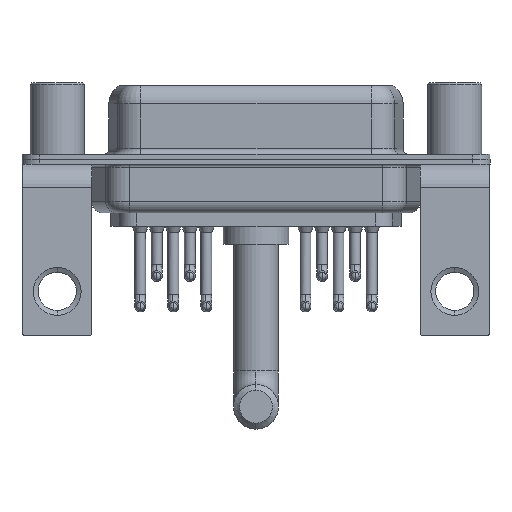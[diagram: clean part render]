
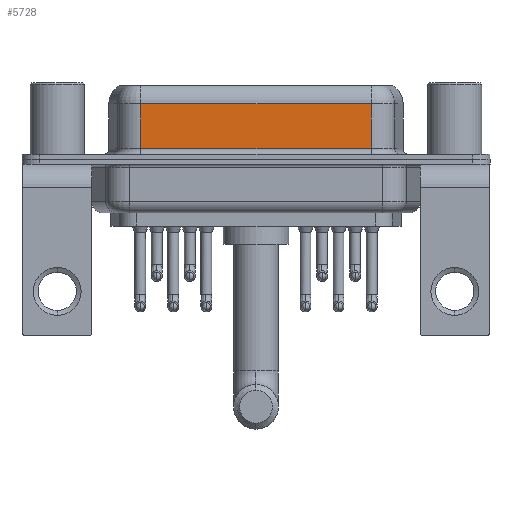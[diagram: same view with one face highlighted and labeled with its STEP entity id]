
A CAD part, front view. The second image highlights one B-rep face of the part: STEP entity #5728.
In plain terms, the highlighted planar face has unit normal (0, -1, 0).
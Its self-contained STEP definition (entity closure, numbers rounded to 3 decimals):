
#185 = LINE ( 'NONE', #8413, #10999 ) ;
#304 = AXIS2_PLACEMENT_3D ( 'NONE', #20353, #5644, #18735 ) ;
#498 = EDGE_CURVE ( 'NONE', #4229, #19295, #185, .T. ) ;
#1807 = CARTESIAN_POINT ( 'NONE',  ( 7.013, -3.95, 4.65 ) ) ;
#2610 = CARTESIAN_POINT ( 'NONE',  ( 26.287, -3.95, 4.65 ) ) ;
#3554 = LINE ( 'NONE', #11489, #19229 ) ;
#4017 = VERTEX_POINT ( 'NONE', #8275 ) ;
#4229 = VERTEX_POINT ( 'NONE', #2610 ) ;
#5076 = CARTESIAN_POINT ( 'NONE',  ( 26.287, -3.95, 4.65 ) ) ;
#5337 = CARTESIAN_POINT ( 'NONE',  ( 7.013, -3.95, 6.4 ) ) ;
#5644 = DIRECTION ( 'NONE',  ( 0., 1., 0. ) ) ;
#5728 = ADVANCED_FACE ( 'NONE', ( #13794 ), #16691, .F. ) ;
#6533 = ORIENTED_EDGE ( 'NONE', *, *, #8854, .T. ) ;
#7129 = DIRECTION ( 'NONE',  ( 0., 0., -1. ) ) ;
#8275 = CARTESIAN_POINT ( 'NONE',  ( 7.013, -3.95, 0.9 ) ) ;
#8380 = EDGE_CURVE ( 'NONE', #4017, #19295, #3554, .T. ) ;
#8413 = CARTESIAN_POINT ( 'NONE',  ( 26.287, -3.95, 6.4 ) ) ;
#8747 = LINE ( 'NONE', #5337, #14789 ) ;
#8854 = EDGE_CURVE ( 'NONE', #17029, #4017, #8747, .T. ) ;
#9869 = DIRECTION ( 'NONE',  ( 1., 0., 0. ) ) ;
#10999 = VECTOR ( 'NONE', #13156, 1000. ) ;
#11027 = ORIENTED_EDGE ( 'NONE', *, *, #8380, .T. ) ;
#11408 = DIRECTION ( 'NONE',  ( -1., 0., 0. ) ) ;
#11489 = CARTESIAN_POINT ( 'NONE',  ( 26.287, -3.95, 0.9 ) ) ;
#12087 = VECTOR ( 'NONE', #11408, 1000. ) ;
#13156 = DIRECTION ( 'NONE',  ( 0., 0., -1. ) ) ;
#13794 = FACE_OUTER_BOUND ( 'NONE', #16971, .T. ) ;
#14310 = ORIENTED_EDGE ( 'NONE', *, *, #19847, .T. ) ;
#14626 = LINE ( 'NONE', #5076, #12087 ) ;
#14789 = VECTOR ( 'NONE', #7129, 1000. ) ;
#16691 = PLANE ( 'NONE',  #304 ) ;
#16971 = EDGE_LOOP ( 'NONE', ( #20632, #14310, #6533, #11027 ) ) ;
#17029 = VERTEX_POINT ( 'NONE', #1807 ) ;
#17364 = CARTESIAN_POINT ( 'NONE',  ( 26.287, -3.95, 0.9 ) ) ;
#18735 = DIRECTION ( 'NONE',  ( 0., 0., 1. ) ) ;
#19229 = VECTOR ( 'NONE', #9869, 1000. ) ;
#19295 = VERTEX_POINT ( 'NONE', #17364 ) ;
#19847 = EDGE_CURVE ( 'NONE', #4229, #17029, #14626, .T. ) ;
#20353 = CARTESIAN_POINT ( 'NONE',  ( 26.287, -3.95, 6.4 ) ) ;
#20632 = ORIENTED_EDGE ( 'NONE', *, *, #498, .F. ) ;
